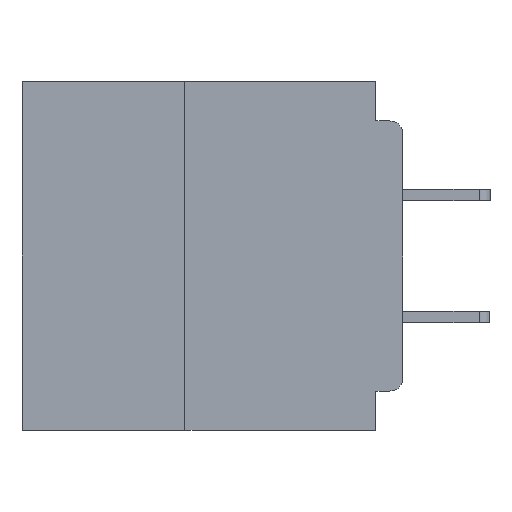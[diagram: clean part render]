
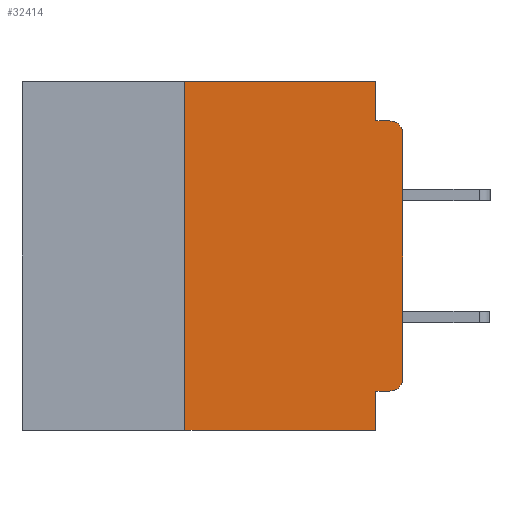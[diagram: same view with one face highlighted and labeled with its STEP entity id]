
A CAD part, left-side view. The second image highlights one B-rep face of the part: STEP entity #32414.
In plain terms, the highlighted planar face has unit normal (-1, 0, 0).
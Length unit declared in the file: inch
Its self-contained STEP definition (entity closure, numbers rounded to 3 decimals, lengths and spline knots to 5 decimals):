
#1161 = CARTESIAN_POINT ( 'NONE',  ( 0., 0.015, -0.045 ) ) ;
#2194 = CIRCLE ( 'NONE', #13520, 0.015 ) ;
#2320 = VERTEX_POINT ( 'NONE', #51661 ) ;
#3089 = EDGE_CURVE ( 'NONE', #49969, #18077, #53578, .T. ) ;
#3437 = VECTOR ( 'NONE', #17361, 39.37008 ) ;
#3987 = EDGE_CURVE ( 'NONE', #11990, #2320, #30369, .T. ) ;
#4220 = EDGE_CURVE ( 'NONE', #21421, #35515, #51845, .T. ) ;
#4420 = VECTOR ( 'NONE', #40233, 39.37008 ) ;
#5475 = LINE ( 'NONE', #25153, #48596 ) ;
#6302 = ORIENTED_EDGE ( 'NONE', *, *, #7327, .T. ) ;
#7327 = EDGE_CURVE ( 'NONE', #15481, #49811, #37757, .T. ) ;
#7591 = ORIENTED_EDGE ( 'NONE', *, *, #3089, .F. ) ;
#7811 = VECTOR ( 'NONE', #37549, 39.37008 ) ;
#8814 = CARTESIAN_POINT ( 'NONE',  ( 0., 0.031, -0.4 ) ) ;
#10237 = CARTESIAN_POINT ( 'NONE',  ( 0., 0., -0.34 ) ) ;
#11325 = PLANE ( 'NONE',  #45769 ) ;
#11990 = VERTEX_POINT ( 'NONE', #10237 ) ;
#13520 = AXIS2_PLACEMENT_3D ( 'NONE', #18751, #47954, #22975 ) ;
#15104 = ORIENTED_EDGE ( 'NONE', *, *, #3987, .T. ) ;
#15481 = VERTEX_POINT ( 'NONE', #51598 ) ;
#15542 = DIRECTION ( 'NONE',  ( 1., 0., 0. ) ) ;
#16032 = ORIENTED_EDGE ( 'NONE', *, *, #53494, .T. ) ;
#16310 = EDGE_CURVE ( 'NONE', #21421, #11990, #46739, .T. ) ;
#16456 = DIRECTION ( 'NONE',  ( -1., 0., 0. ) ) ;
#17361 = DIRECTION ( 'NONE',  ( 0., 0., -1. ) ) ;
#18077 = VERTEX_POINT ( 'NONE', #1161 ) ;
#18546 = VECTOR ( 'NONE', #28180, 39.37008 ) ;
#18751 = CARTESIAN_POINT ( 'NONE',  ( 0., 0.015, -0.06 ) ) ;
#18853 = LINE ( 'NONE', #8814, #28683 ) ;
#19547 = CARTESIAN_POINT ( 'NONE',  ( 0., 0.031, -0.045 ) ) ;
#20415 = EDGE_CURVE ( 'NONE', #35515, #49811, #18853, .T. ) ;
#21235 = DIRECTION ( 'NONE',  ( 0., 0., 1. ) ) ;
#21421 = VERTEX_POINT ( 'NONE', #29696 ) ;
#22975 = DIRECTION ( 'NONE',  ( 0., 0., -1. ) ) ;
#24424 = EDGE_CURVE ( 'NONE', #15481, #31843, #48184, .T. ) ;
#25153 = CARTESIAN_POINT ( 'NONE',  ( 0., 0.437, 0. ) ) ;
#25511 = DIRECTION ( 'NONE',  ( 0., 0., -1. ) ) ;
#25696 = EDGE_CURVE ( 'NONE', #31843, #31035, #5475, .T. ) ;
#25839 = ORIENTED_EDGE ( 'NONE', *, *, #24424, .F. ) ;
#26105 = ORIENTED_EDGE ( 'NONE', *, *, #25696, .F. ) ;
#26409 = ORIENTED_EDGE ( 'NONE', *, *, #20415, .F. ) ;
#27284 = EDGE_LOOP ( 'NONE', ( #15104, #16032, #7591, #36541, #26105, #25839, #6302, #26409, #35712, #28738 ) ) ;
#27316 = CARTESIAN_POINT ( 'NONE',  ( 0., 0.031, -0.355 ) ) ;
#27448 = AXIS2_PLACEMENT_3D ( 'NONE', #41473, #16456, #45681 ) ;
#28180 = DIRECTION ( 'NONE',  ( 0., 1., 0. ) ) ;
#28642 = CARTESIAN_POINT ( 'NONE',  ( 0., 0.031, 0. ) ) ;
#28683 = VECTOR ( 'NONE', #25511, 39.37008 ) ;
#28738 = ORIENTED_EDGE ( 'NONE', *, *, #16310, .T. ) ;
#29219 = CARTESIAN_POINT ( 'NONE',  ( 0., 0., -0.045 ) ) ;
#29373 = DIRECTION ( 'NONE',  ( 0., -1., 0. ) ) ;
#29696 = CARTESIAN_POINT ( 'NONE',  ( 0., 0.015, -0.355 ) ) ;
#30369 = LINE ( 'NONE', #43111, #51209 ) ;
#30936 = CARTESIAN_POINT ( 'NONE',  ( 0., 0.031, -0.4 ) ) ;
#31035 = VERTEX_POINT ( 'NONE', #28642 ) ;
#31843 = VERTEX_POINT ( 'NONE', #34932 ) ;
#32414 = ADVANCED_FACE ( 'NONE', ( #47796 ), #11325, .F. ) ;
#34932 = CARTESIAN_POINT ( 'NONE',  ( 0., 0.25, 0. ) ) ;
#35515 = VERTEX_POINT ( 'NONE', #27316 ) ;
#35712 = ORIENTED_EDGE ( 'NONE', *, *, #4220, .F. ) ;
#36065 = CARTESIAN_POINT ( 'NONE',  ( 0., 0.437, -0.4 ) ) ;
#36541 = ORIENTED_EDGE ( 'NONE', *, *, #40716, .F. ) ;
#36825 = LINE ( 'NONE', #46552, #3437 ) ;
#37549 = DIRECTION ( 'NONE',  ( 0., -1., 0. ) ) ;
#37757 = LINE ( 'NONE', #36065, #4420 ) ;
#40233 = DIRECTION ( 'NONE',  ( 0., -1., 0. ) ) ;
#40716 = EDGE_CURVE ( 'NONE', #31035, #49969, #36825, .T. ) ;
#41473 = CARTESIAN_POINT ( 'NONE',  ( 0., 0.015, -0.34 ) ) ;
#43111 = CARTESIAN_POINT ( 'NONE',  ( 0., 0., 0. ) ) ;
#44741 = DIRECTION ( 'NONE',  ( 0., 0., -1. ) ) ;
#45562 = VECTOR ( 'NONE', #21235, 39.37008 ) ;
#45681 = DIRECTION ( 'NONE',  ( 0., 0., -1. ) ) ;
#45769 = AXIS2_PLACEMENT_3D ( 'NONE', #52955, #15542, #44741 ) ;
#46552 = CARTESIAN_POINT ( 'NONE',  ( 0., 0.031, 0. ) ) ;
#46739 = CIRCLE ( 'NONE', #27448, 0.015 ) ;
#47796 = FACE_OUTER_BOUND ( 'NONE', #27284, .T. ) ;
#47954 = DIRECTION ( 'NONE',  ( -1., 0., 0. ) ) ;
#48184 = LINE ( 'NONE', #50418, #45562 ) ;
#48596 = VECTOR ( 'NONE', #29373, 39.37008 ) ;
#49811 = VERTEX_POINT ( 'NONE', #30936 ) ;
#49969 = VERTEX_POINT ( 'NONE', #19547 ) ;
#50418 = CARTESIAN_POINT ( 'NONE',  ( 0., 0.25, -0.4 ) ) ;
#51209 = VECTOR ( 'NONE', #51516, 39.37008 ) ;
#51516 = DIRECTION ( 'NONE',  ( 0., 0., 1. ) ) ;
#51598 = CARTESIAN_POINT ( 'NONE',  ( 0., 0.25, -0.4 ) ) ;
#51661 = CARTESIAN_POINT ( 'NONE',  ( 0., 0., -0.06 ) ) ;
#51845 = LINE ( 'NONE', #53148, #18546 ) ;
#52955 = CARTESIAN_POINT ( 'NONE',  ( 0., 0.437, 0. ) ) ;
#53148 = CARTESIAN_POINT ( 'NONE',  ( 0., 0., -0.355 ) ) ;
#53494 = EDGE_CURVE ( 'NONE', #2320, #18077, #2194, .T. ) ;
#53578 = LINE ( 'NONE', #29219, #7811 ) ;
